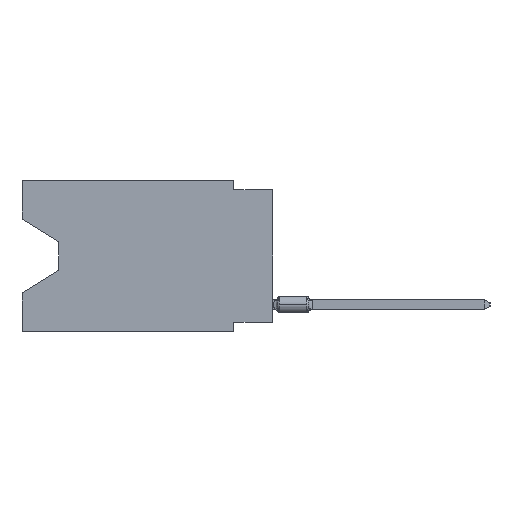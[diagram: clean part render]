
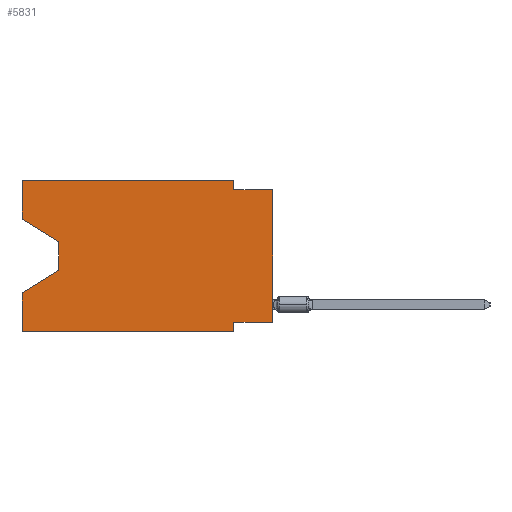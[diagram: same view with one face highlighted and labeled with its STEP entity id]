
A CAD part, left-side view. The second image highlights one B-rep face of the part: STEP entity #5831.
In plain terms, the highlighted planar face has unit normal (-1, 0, 0).
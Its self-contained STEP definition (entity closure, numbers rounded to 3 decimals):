
#1239 = ORIENTED_EDGE ( 'NONE', *, *, #39699, .T. ) ;
#2480 = VECTOR ( 'NONE', #83809, 1000. ) ;
#2863 = ORIENTED_EDGE ( 'NONE', *, *, #11783, .F. ) ;
#3113 = CARTESIAN_POINT ( 'NONE',  ( 0., 2.54, -0.635 ) ) ;
#3237 = DIRECTION ( 'NONE',  ( 0., 0., 1. ) ) ;
#4352 = VECTOR ( 'NONE', #79538, 1000. ) ;
#5240 = ORIENTED_EDGE ( 'NONE', *, *, #52373, .F. ) ;
#5831 = ADVANCED_FACE ( 'NONE', ( #13961 ), #74934, .F. ) ;
#6513 = CARTESIAN_POINT ( 'NONE',  ( 0., 16.383, 0. ) ) ;
#6939 = VERTEX_POINT ( 'NONE', #64143 ) ;
#11401 = CARTESIAN_POINT ( 'NONE',  ( 0., 2.54, -9.906 ) ) ;
#11783 = EDGE_CURVE ( 'NONE', #6939, #77036, #32153, .T. ) ;
#12073 = CARTESIAN_POINT ( 'NONE',  ( 0., 16.383, -9.906 ) ) ;
#13961 = FACE_OUTER_BOUND ( 'NONE', #68726, .T. ) ;
#14820 = DIRECTION ( 'NONE',  ( 1., 0., 0. ) ) ;
#15417 = LINE ( 'NONE', #67650, #64068 ) ;
#15451 = ORIENTED_EDGE ( 'NONE', *, *, #17636, .T. ) ;
#15757 = LINE ( 'NONE', #75878, #51873 ) ;
#16693 = VECTOR ( 'NONE', #72169, 1000. ) ;
#16987 = CARTESIAN_POINT ( 'NONE',  ( 0., 0., -0.635 ) ) ;
#17636 = EDGE_CURVE ( 'NONE', #83332, #22973, #31794, .T. ) ;
#19983 = VERTEX_POINT ( 'NONE', #51550 ) ;
#20688 = EDGE_CURVE ( 'NONE', #78357, #50611, #15417, .T. ) ;
#22973 = VERTEX_POINT ( 'NONE', #40788 ) ;
#23844 = CARTESIAN_POINT ( 'NONE',  ( 0., 16.383, -7.36 ) ) ;
#24198 = VECTOR ( 'NONE', #60462, 1000. ) ;
#24290 = CARTESIAN_POINT ( 'NONE',  ( 0., 0., -9.271 ) ) ;
#25820 = EDGE_CURVE ( 'NONE', #67730, #30310, #44310, .T. ) ;
#27985 = LINE ( 'NONE', #53445, #24198 ) ;
#30088 = VECTOR ( 'NONE', #77830, 1000. ) ;
#30310 = VERTEX_POINT ( 'NONE', #64800 ) ;
#30950 = ORIENTED_EDGE ( 'NONE', *, *, #20688, .T. ) ;
#31373 = ORIENTED_EDGE ( 'NONE', *, *, #40682, .T. ) ;
#31794 = LINE ( 'NONE', #39235, #16693 ) ;
#32153 = LINE ( 'NONE', #24290, #30088 ) ;
#35002 = LINE ( 'NONE', #60048, #63409 ) ;
#35602 = ORIENTED_EDGE ( 'NONE', *, *, #60337, .F. ) ;
#36230 = VERTEX_POINT ( 'NONE', #54744 ) ;
#39235 = CARTESIAN_POINT ( 'NONE',  ( 0., 16.383, -2.546 ) ) ;
#39593 = CARTESIAN_POINT ( 'NONE',  ( 0., 13.97, -4.013 ) ) ;
#39699 = EDGE_CURVE ( 'NONE', #6939, #19983, #15757, .T. ) ;
#40682 = EDGE_CURVE ( 'NONE', #22973, #78357, #52760, .T. ) ;
#40788 = CARTESIAN_POINT ( 'NONE',  ( 0., 13.97, -4.013 ) ) ;
#42172 = DIRECTION ( 'NONE',  ( 0., 0.855, -0.519 ) ) ;
#42695 = CARTESIAN_POINT ( 'NONE',  ( 0., 2.54, -9.271 ) ) ;
#43928 = LINE ( 'NONE', #73294, #70447 ) ;
#44310 = LINE ( 'NONE', #63628, #69314 ) ;
#44585 = CARTESIAN_POINT ( 'NONE',  ( 0., 16.383, -2.546 ) ) ;
#44884 = ORIENTED_EDGE ( 'NONE', *, *, #25820, .T. ) ;
#48016 = ORIENTED_EDGE ( 'NONE', *, *, #71226, .F. ) ;
#49518 = DIRECTION ( 'NONE',  ( 0., 0., 1. ) ) ;
#49927 = VECTOR ( 'NONE', #58629, 1000. ) ;
#50611 = VERTEX_POINT ( 'NONE', #23844 ) ;
#51550 = CARTESIAN_POINT ( 'NONE',  ( 0., 0., -0.635 ) ) ;
#51873 = VECTOR ( 'NONE', #49518, 1000. ) ;
#52373 = EDGE_CURVE ( 'NONE', #83332, #36230, #43928, .T. ) ;
#52760 = LINE ( 'NONE', #39593, #4352 ) ;
#53277 = AXIS2_PLACEMENT_3D ( 'NONE', #6513, #14820, #73641 ) ;
#53445 = CARTESIAN_POINT ( 'NONE',  ( 0., 16.383, 0. ) ) ;
#53776 = ORIENTED_EDGE ( 'NONE', *, *, #72479, .F. ) ;
#53924 = VERTEX_POINT ( 'NONE', #78560 ) ;
#54478 = ORIENTED_EDGE ( 'NONE', *, *, #77542, .F. ) ;
#54744 = CARTESIAN_POINT ( 'NONE',  ( 0., 16.383, 0. ) ) ;
#56582 = EDGE_CURVE ( 'NONE', #67730, #50611, #70785, .T. ) ;
#58629 = DIRECTION ( 'NONE',  ( 0., -1., 0. ) ) ;
#58791 = ORIENTED_EDGE ( 'NONE', *, *, #56582, .F. ) ;
#60048 = CARTESIAN_POINT ( 'NONE',  ( 0., 2.54, 0. ) ) ;
#60337 = EDGE_CURVE ( 'NONE', #77036, #30310, #64509, .T. ) ;
#60462 = DIRECTION ( 'NONE',  ( 0., -1., 0. ) ) ;
#63205 = DIRECTION ( 'NONE',  ( 0., -1., 0. ) ) ;
#63409 = VECTOR ( 'NONE', #83456, 1000. ) ;
#63628 = CARTESIAN_POINT ( 'NONE',  ( 0., 16.383, -9.906 ) ) ;
#64068 = VECTOR ( 'NONE', #42172, 1000. ) ;
#64143 = CARTESIAN_POINT ( 'NONE',  ( 0., 0., -9.271 ) ) ;
#64198 = CARTESIAN_POINT ( 'NONE',  ( 0., 16.383, 0. ) ) ;
#64509 = LINE ( 'NONE', #11401, #2480 ) ;
#64800 = CARTESIAN_POINT ( 'NONE',  ( 0., 2.54, -9.906 ) ) ;
#66874 = VERTEX_POINT ( 'NONE', #3113 ) ;
#67650 = CARTESIAN_POINT ( 'NONE',  ( 0., 13.97, -5.893 ) ) ;
#67730 = VERTEX_POINT ( 'NONE', #12073 ) ;
#68726 = EDGE_LOOP ( 'NONE', ( #15451, #31373, #30950, #58791, #44884, #35602, #2863, #1239, #54478, #53776, #48016, #5240 ) ) ;
#69314 = VECTOR ( 'NONE', #63205, 1000. ) ;
#70447 = VECTOR ( 'NONE', #85586, 1000. ) ;
#70785 = LINE ( 'NONE', #64198, #80769 ) ;
#71226 = EDGE_CURVE ( 'NONE', #36230, #53924, #27985, .T. ) ;
#72169 = DIRECTION ( 'NONE',  ( 0., -0.855, -0.519 ) ) ;
#72479 = EDGE_CURVE ( 'NONE', #53924, #66874, #35002, .T. ) ;
#73294 = CARTESIAN_POINT ( 'NONE',  ( 0., 16.383, 0. ) ) ;
#73641 = DIRECTION ( 'NONE',  ( 0., 0., -1. ) ) ;
#74089 = CARTESIAN_POINT ( 'NONE',  ( 0., 13.97, -5.893 ) ) ;
#74934 = PLANE ( 'NONE',  #53277 ) ;
#75878 = CARTESIAN_POINT ( 'NONE',  ( 0., 0., 0. ) ) ;
#77036 = VERTEX_POINT ( 'NONE', #42695 ) ;
#77100 = LINE ( 'NONE', #16987, #49927 ) ;
#77542 = EDGE_CURVE ( 'NONE', #66874, #19983, #77100, .T. ) ;
#77830 = DIRECTION ( 'NONE',  ( 0., 1., 0. ) ) ;
#78357 = VERTEX_POINT ( 'NONE', #74089 ) ;
#78560 = CARTESIAN_POINT ( 'NONE',  ( 0., 2.54, 0. ) ) ;
#79538 = DIRECTION ( 'NONE',  ( 0., 0., -1. ) ) ;
#80769 = VECTOR ( 'NONE', #3237, 1000. ) ;
#83332 = VERTEX_POINT ( 'NONE', #44585 ) ;
#83456 = DIRECTION ( 'NONE',  ( 0., 0., -1. ) ) ;
#83809 = DIRECTION ( 'NONE',  ( 0., 0., -1. ) ) ;
#85586 = DIRECTION ( 'NONE',  ( 0., 0., 1. ) ) ;
